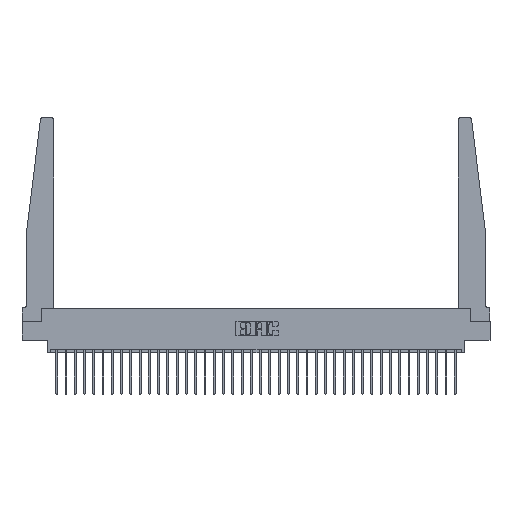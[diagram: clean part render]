
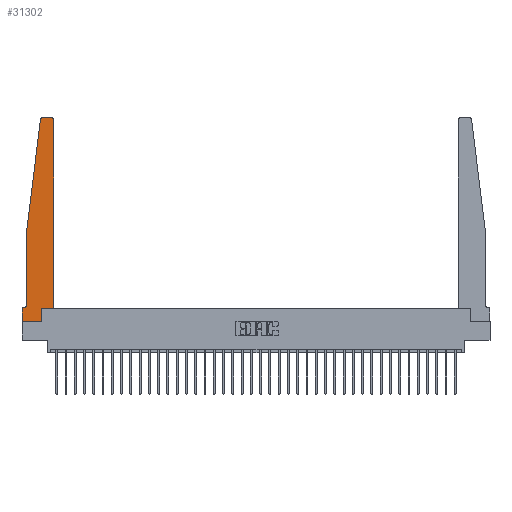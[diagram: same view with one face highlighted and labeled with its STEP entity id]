
A CAD part, top view. The second image highlights one B-rep face of the part: STEP entity #31302.
In plain terms, the highlighted planar face has unit normal (0, 0, 1).
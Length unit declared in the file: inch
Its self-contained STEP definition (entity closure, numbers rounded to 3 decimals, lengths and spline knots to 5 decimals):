
#41 = CARTESIAN_POINT ( 'NONE',  ( 0.425, 0.18, 0.37 ) ) ;
#343 = CARTESIAN_POINT ( 'NONE',  ( 0.395, 2.75, 0.37 ) ) ;
#542 = CIRCLE ( 'NONE', #8718, 0.05 ) ;
#628 = EDGE_CURVE ( 'NONE', #11729, #2941, #28550, .T. ) ;
#1515 = CARTESIAN_POINT ( 'NONE',  ( 0., 0.1875, 0.37 ) ) ;
#1608 = VERTEX_POINT ( 'NONE', #41 ) ;
#1666 = CARTESIAN_POINT ( 'NONE',  ( 0.065, 1.25, 0.37 ) ) ;
#1688 = VERTEX_POINT ( 'NONE', #26702 ) ;
#2221 = ORIENTED_EDGE ( 'NONE', *, *, #4294, .T. ) ;
#2229 = AXIS2_PLACEMENT_3D ( 'NONE', #1515, #22388, #22220 ) ;
#2783 = VECTOR ( 'NONE', #5124, 39.37008 ) ;
#2879 = DIRECTION ( 'NONE',  ( 1., 0., 0. ) ) ;
#2941 = VERTEX_POINT ( 'NONE', #22107 ) ;
#3088 = ORIENTED_EDGE ( 'NONE', *, *, #9781, .T. ) ;
#3736 = CARTESIAN_POINT ( 'NONE',  ( 0., 0.1875, 0.37 ) ) ;
#4092 = LINE ( 'NONE', #6656, #25820 ) ;
#4132 = CARTESIAN_POINT ( 'NONE',  ( 0.27653, 2.72, 0.37 ) ) ;
#4212 = DIRECTION ( 'NONE',  ( 0., -1., 0. ) ) ;
#4294 = EDGE_CURVE ( 'NONE', #2941, #25950, #6473, .T. ) ;
#4407 = DIRECTION ( 'NONE',  ( 0., -1., 0. ) ) ;
#4428 = AXIS2_PLACEMENT_3D ( 'NONE', #26521, #5468, #29249 ) ;
#4457 = ORIENTED_EDGE ( 'NONE', *, *, #5465, .T. ) ;
#4650 = DIRECTION ( 'NONE',  ( 0., 0., 1. ) ) ;
#4654 = VERTEX_POINT ( 'NONE', #3736 ) ;
#4821 = ORIENTED_EDGE ( 'NONE', *, *, #10598, .T. ) ;
#4903 = VERTEX_POINT ( 'NONE', #20653 ) ;
#5124 = DIRECTION ( 'NONE',  ( -1., 0., 0. ) ) ;
#5465 = EDGE_CURVE ( 'NONE', #1688, #8426, #542, .T. ) ;
#5468 = DIRECTION ( 'NONE',  ( 0., 0., 1. ) ) ;
#5554 = CARTESIAN_POINT ( 'NONE',  ( 0.065, 1.25, 0.37 ) ) ;
#5610 = EDGE_CURVE ( 'NONE', #4903, #16603, #32050, .T. ) ;
#6162 = LINE ( 'NONE', #27025, #32082 ) ;
#6473 = CIRCLE ( 'NONE', #32127, 0.03 ) ;
#6656 = CARTESIAN_POINT ( 'NONE',  ( 0.425, 0.18, 0.37 ) ) ;
#6729 = VERTEX_POINT ( 'NONE', #5554 ) ;
#6742 = DIRECTION ( 'NONE',  ( 0., 0., -1. ) ) ;
#6959 = CARTESIAN_POINT ( 'NONE',  ( 0.065, 1.25, 0.37 ) ) ;
#7871 = ORIENTED_EDGE ( 'NONE', *, *, #628, .T. ) ;
#7917 = EDGE_CURVE ( 'NONE', #8426, #4654, #6162, .T. ) ;
#8334 = EDGE_CURVE ( 'NONE', #15993, #4903, #21346, .T. ) ;
#8426 = VERTEX_POINT ( 'NONE', #10302 ) ;
#8609 = VECTOR ( 'NONE', #4212, 39.37008 ) ;
#8718 = AXIS2_PLACEMENT_3D ( 'NONE', #19758, #6742, #17180 ) ;
#9781 = EDGE_CURVE ( 'NONE', #25950, #6729, #25428, .T. ) ;
#10302 = CARTESIAN_POINT ( 'NONE',  ( 0.015, 0.1875, 0.37 ) ) ;
#10598 = EDGE_CURVE ( 'NONE', #4654, #15993, #19471, .T. ) ;
#10969 = ORIENTED_EDGE ( 'NONE', *, *, #30393, .T. ) ;
#11466 = ORIENTED_EDGE ( 'NONE', *, *, #8334, .T. ) ;
#11729 = VERTEX_POINT ( 'NONE', #343 ) ;
#11789 = PLANE ( 'NONE',  #2229 ) ;
#12875 = ORIENTED_EDGE ( 'NONE', *, *, #14821, .T. ) ;
#13680 = EDGE_CURVE ( 'NONE', #6729, #1688, #33498, .T. ) ;
#13815 = ORIENTED_EDGE ( 'NONE', *, *, #13680, .T. ) ;
#14040 = ORIENTED_EDGE ( 'NONE', *, *, #32956, .T. ) ;
#14568 = VECTOR ( 'NONE', #29551, 39.37008 ) ;
#14821 = EDGE_CURVE ( 'NONE', #16603, #1608, #16207, .T. ) ;
#15993 = VERTEX_POINT ( 'NONE', #16213 ) ;
#16207 = LINE ( 'NONE', #16560, #18091 ) ;
#16213 = CARTESIAN_POINT ( 'NONE',  ( 0., 0., 0.37 ) ) ;
#16560 = CARTESIAN_POINT ( 'NONE',  ( 0.425, 0.18, 0.37 ) ) ;
#16603 = VERTEX_POINT ( 'NONE', #25243 ) ;
#17090 = DIRECTION ( 'NONE',  ( 0., 1., 0. ) ) ;
#17180 = DIRECTION ( 'NONE',  ( -1., 0., 0. ) ) ;
#17403 = DIRECTION ( 'NONE',  ( -0.122, -0.992, 0. ) ) ;
#18091 = VECTOR ( 'NONE', #2879, 39.37008 ) ;
#19471 = LINE ( 'NONE', #25425, #8609 ) ;
#19674 = FACE_OUTER_BOUND ( 'NONE', #31073, .T. ) ;
#19758 = CARTESIAN_POINT ( 'NONE',  ( 0.015, 0.2375, 0.37 ) ) ;
#20594 = ORIENTED_EDGE ( 'NONE', *, *, #7917, .T. ) ;
#20653 = CARTESIAN_POINT ( 'NONE',  ( 0.2605, 0., 0.37 ) ) ;
#21346 = LINE ( 'NONE', #21664, #14568 ) ;
#21664 = CARTESIAN_POINT ( 'NONE',  ( 0., 0., 0.37 ) ) ;
#22107 = CARTESIAN_POINT ( 'NONE',  ( 0.27653, 2.75, 0.37 ) ) ;
#22220 = DIRECTION ( 'NONE',  ( 1., 0., 0. ) ) ;
#22295 = CARTESIAN_POINT ( 'NONE',  ( 0.2605, 0.18, 0.37 ) ) ;
#22388 = DIRECTION ( 'NONE',  ( 0., 0., 1. ) ) ;
#23491 = VECTOR ( 'NONE', #4407, 39.37008 ) ;
#25184 = CIRCLE ( 'NONE', #4428, 0.03 ) ;
#25243 = CARTESIAN_POINT ( 'NONE',  ( 0.2605, 0.18, 0.37 ) ) ;
#25425 = CARTESIAN_POINT ( 'NONE',  ( 0., 0., 0.37 ) ) ;
#25428 = LINE ( 'NONE', #1666, #30897 ) ;
#25495 = DIRECTION ( 'NONE',  ( 1., 0., 0. ) ) ;
#25820 = VECTOR ( 'NONE', #17090, 39.37008 ) ;
#25950 = VERTEX_POINT ( 'NONE', #30436 ) ;
#26521 = CARTESIAN_POINT ( 'NONE',  ( 0.395, 2.72, 0.37 ) ) ;
#26702 = CARTESIAN_POINT ( 'NONE',  ( 0.065, 0.2375, 0.37 ) ) ;
#27025 = CARTESIAN_POINT ( 'NONE',  ( 0.065, 0.1875, 0.37 ) ) ;
#27090 = DIRECTION ( 'NONE',  ( 0., 1., 0. ) ) ;
#27870 = CARTESIAN_POINT ( 'NONE',  ( 0.25, 2.75, 0.37 ) ) ;
#28393 = ORIENTED_EDGE ( 'NONE', *, *, #5610, .T. ) ;
#28550 = LINE ( 'NONE', #27870, #2783 ) ;
#29249 = DIRECTION ( 'NONE',  ( 1., 0., 0. ) ) ;
#29551 = DIRECTION ( 'NONE',  ( 1., 0., 0. ) ) ;
#29752 = DIRECTION ( 'NONE',  ( -1., 0., 0. ) ) ;
#30393 = EDGE_CURVE ( 'NONE', #1608, #32726, #4092, .T. ) ;
#30436 = CARTESIAN_POINT ( 'NONE',  ( 0.24675, 2.72367, 0.37 ) ) ;
#30897 = VECTOR ( 'NONE', #17403, 39.37008 ) ;
#31073 = EDGE_LOOP ( 'NONE', ( #7871, #2221, #3088, #13815, #4457, #20594, #4821, #11466, #28393, #12875, #10969, #14040 ) ) ;
#31302 = ADVANCED_FACE ( 'NONE', ( #19674 ), #11789, .T. ) ;
#31664 = VECTOR ( 'NONE', #27090, 39.37008 ) ;
#32050 = LINE ( 'NONE', #22295, #31664 ) ;
#32082 = VECTOR ( 'NONE', #29752, 39.37008 ) ;
#32127 = AXIS2_PLACEMENT_3D ( 'NONE', #4132, #4650, #25495 ) ;
#32726 = VERTEX_POINT ( 'NONE', #33209 ) ;
#32956 = EDGE_CURVE ( 'NONE', #32726, #11729, #25184, .T. ) ;
#33209 = CARTESIAN_POINT ( 'NONE',  ( 0.425, 2.72, 0.37 ) ) ;
#33498 = LINE ( 'NONE', #6959, #23491 ) ;
